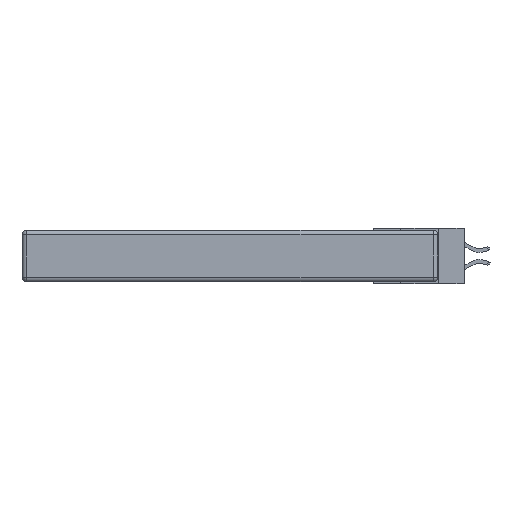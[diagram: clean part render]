
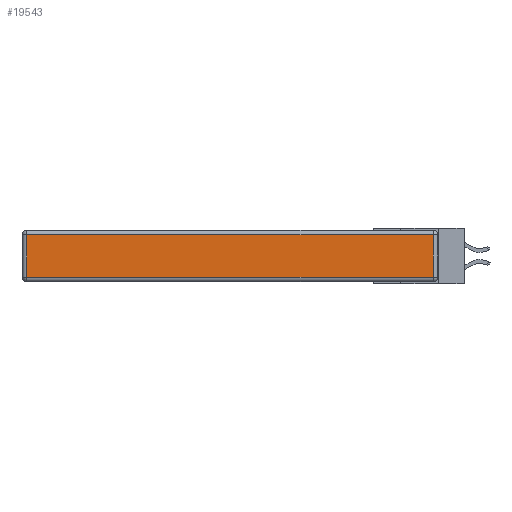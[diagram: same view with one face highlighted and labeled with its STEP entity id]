
A CAD part, left-side view. The second image highlights one B-rep face of the part: STEP entity #19543.
In plain terms, the highlighted planar face has unit normal (-1, 0, 0).
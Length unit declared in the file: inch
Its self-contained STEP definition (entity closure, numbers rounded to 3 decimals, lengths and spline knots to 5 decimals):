
#120 = LINE ( 'NONE', #6585, #9821 ) ;
#505 = DIRECTION ( 'NONE',  ( 0., 0., 1. ) ) ;
#575 = CARTESIAN_POINT ( 'NONE',  ( 0., 0.03, -0.343 ) ) ;
#774 = AXIS2_PLACEMENT_3D ( 'NONE', #7115, #5702, #8684 ) ;
#1051 = ORIENTED_EDGE ( 'NONE', *, *, #11611, .T. ) ;
#1063 = VECTOR ( 'NONE', #6817, 39.37008 ) ;
#1523 = CARTESIAN_POINT ( 'NONE',  ( 0., 0.03, -0.03 ) ) ;
#2521 = CARTESIAN_POINT ( 'NONE',  ( 0., 2.72, -0.313 ) ) ;
#2560 = PLANE ( 'NONE',  #774 ) ;
#2572 = EDGE_CURVE ( 'NONE', #19890, #18823, #18481, .T. ) ;
#2999 = ORIENTED_EDGE ( 'NONE', *, *, #3952, .T. ) ;
#3378 = VECTOR ( 'NONE', #505, 39.37008 ) ;
#3952 = EDGE_CURVE ( 'NONE', #18823, #11649, #4204, .T. ) ;
#4204 = LINE ( 'NONE', #14447, #1063 ) ;
#4308 = DIRECTION ( 'NONE',  ( 0., -1., 0. ) ) ;
#4342 = CARTESIAN_POINT ( 'NONE',  ( 0., 0.03, -0.313 ) ) ;
#5489 = EDGE_LOOP ( 'NONE', ( #12877, #6321, #2999, #1051 ) ) ;
#5702 = DIRECTION ( 'NONE',  ( -1., 0., 0. ) ) ;
#5758 = CARTESIAN_POINT ( 'NONE',  ( 0., 0., -0.313 ) ) ;
#6308 = DIRECTION ( 'NONE',  ( 0., 0., -1. ) ) ;
#6321 = ORIENTED_EDGE ( 'NONE', *, *, #2572, .T. ) ;
#6585 = CARTESIAN_POINT ( 'NONE',  ( 0., 2.72, -0.343 ) ) ;
#6817 = DIRECTION ( 'NONE',  ( 0., 1., 0. ) ) ;
#7115 = CARTESIAN_POINT ( 'NONE',  ( 0., 0., -0.343 ) ) ;
#8684 = DIRECTION ( 'NONE',  ( 0., 0., 1. ) ) ;
#9813 = EDGE_CURVE ( 'NONE', #17190, #19890, #13960, .T. ) ;
#9821 = VECTOR ( 'NONE', #6308, 39.37008 ) ;
#10838 = VECTOR ( 'NONE', #4308, 39.37008 ) ;
#11611 = EDGE_CURVE ( 'NONE', #11649, #17190, #120, .T. ) ;
#11649 = VERTEX_POINT ( 'NONE', #12575 ) ;
#12575 = CARTESIAN_POINT ( 'NONE',  ( 0., 2.72, -0.03 ) ) ;
#12877 = ORIENTED_EDGE ( 'NONE', *, *, #9813, .T. ) ;
#13960 = LINE ( 'NONE', #5758, #10838 ) ;
#14447 = CARTESIAN_POINT ( 'NONE',  ( 0., 2.75, -0.03 ) ) ;
#17190 = VERTEX_POINT ( 'NONE', #2521 ) ;
#17910 = FACE_OUTER_BOUND ( 'NONE', #5489, .T. ) ;
#18481 = LINE ( 'NONE', #575, #3378 ) ;
#18823 = VERTEX_POINT ( 'NONE', #1523 ) ;
#19543 = ADVANCED_FACE ( 'NONE', ( #17910 ), #2560, .T. ) ;
#19890 = VERTEX_POINT ( 'NONE', #4342 ) ;
